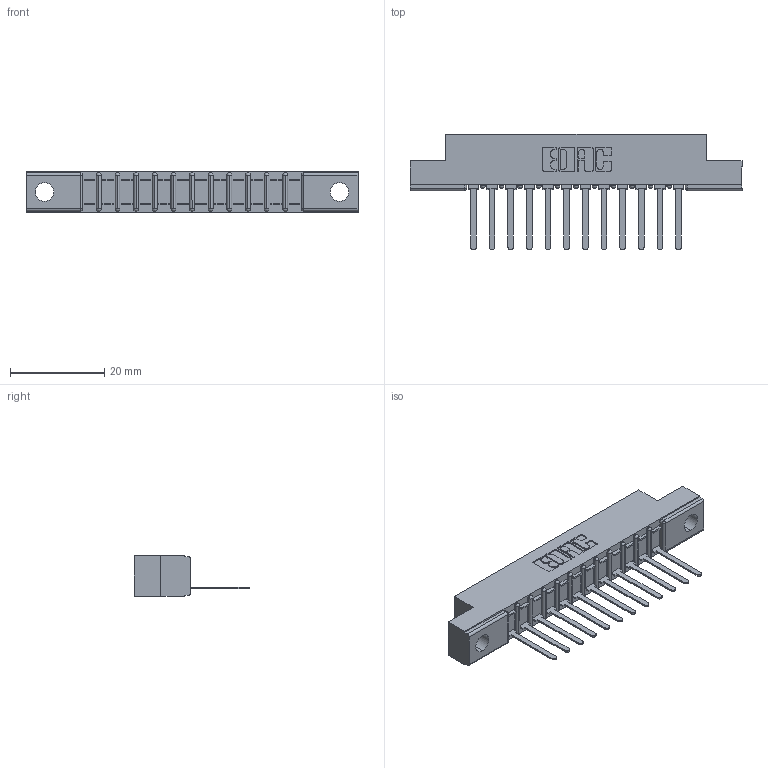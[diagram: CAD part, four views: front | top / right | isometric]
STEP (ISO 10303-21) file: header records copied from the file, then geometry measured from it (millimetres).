
FILE_DESCRIPTION (( 'STEP AP203' ), '1' );
FILE_NAME ('307-012-441-104.STEP', '2020-09-25T12:11:41', ( '' ), ( '' ), 'SwSTEP 2.0', 'SolidWorks 2020', '' );
FILE_SCHEMA (( 'CONFIG_CONTROL_DESIGN' ));
Length unit declared in the file: inch
Products named in the file (3): 307-290-002_541; 307 Part_.156 Dia Mounting Holes; 307-012-441-104
Assembly tree (13 placements, depth 2):
  307-012-441-104
    307 Part_.156 Dia Mounting Holes
    307-290-002_541  x12
Bounding box: 70.56 x 24.59 x 8.71 mm (x, y, z)
Volume: 4581 mm3; surface area: 7871.3 mm2
Topology: 13 solids, 13 shells, 1033 faces, 3143 edges, 2058 vertices
Faces by surface type: plane 624, cylinder 383, sphere 26
Entity records: 15122 total; most frequent: CARTESIAN_POINT 2550, ORIENTED_EDGE 2538, DIRECTION 2483, EDGE_CURVE 1269, LINE 965, VECTOR 965, VERTEX_POINT 826, AXIS2_PLACEMENT_3D 759
